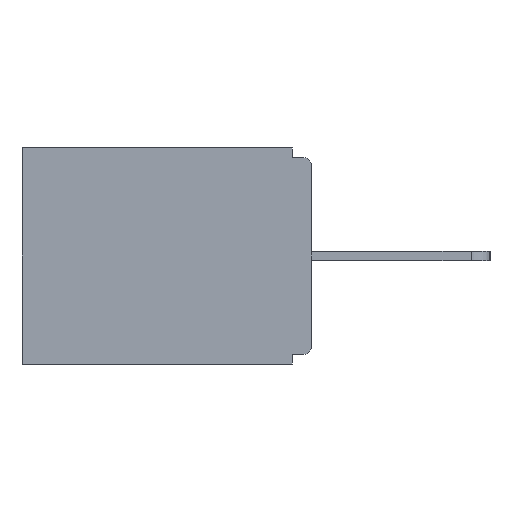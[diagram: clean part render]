
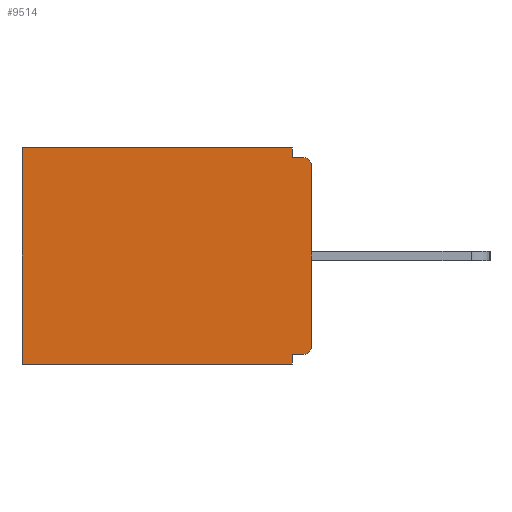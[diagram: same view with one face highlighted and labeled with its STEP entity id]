
A CAD part, left-side view. The second image highlights one B-rep face of the part: STEP entity #9514.
In plain terms, the highlighted planar face has unit normal (-1, 0, 0).
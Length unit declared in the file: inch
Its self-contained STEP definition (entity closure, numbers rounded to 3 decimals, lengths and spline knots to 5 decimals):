
#617 = VECTOR ( 'NONE', #4318, 39.37008 ) ;
#638 = CARTESIAN_POINT ( 'NONE',  ( 0.298, 0.015, -0.015 ) ) ;
#838 = EDGE_CURVE ( 'NONE', #17202, #10318, #16039, .T. ) ;
#1009 = ORIENTED_EDGE ( 'NONE', *, *, #4392, .F. ) ;
#1059 = CARTESIAN_POINT ( 'NONE',  ( 0.298, 0., -0.328 ) ) ;
#1076 = ORIENTED_EDGE ( 'NONE', *, *, #10512, .T. ) ;
#1226 = DIRECTION ( 'NONE',  ( 0., 0., -1. ) ) ;
#1297 = CARTESIAN_POINT ( 'NONE',  ( 0.298, 0.015, -0.03 ) ) ;
#1445 = CARTESIAN_POINT ( 'NONE',  ( 0.298, 0.015, -0.328 ) ) ;
#1468 = VERTEX_POINT ( 'NONE', #1445 ) ;
#1560 = EDGE_CURVE ( 'NONE', #2902, #17478, #16222, .T. ) ;
#1816 = DIRECTION ( 'NONE',  ( -1., 0., 0. ) ) ;
#1899 = ORIENTED_EDGE ( 'NONE', *, *, #18720, .T. ) ;
#2090 = CARTESIAN_POINT ( 'NONE',  ( 0.298, 0., -0.03 ) ) ;
#2370 = FACE_OUTER_BOUND ( 'NONE', #15454, .T. ) ;
#2758 = CARTESIAN_POINT ( 'NONE',  ( 0.298, 0.031, -0.015 ) ) ;
#2902 = VERTEX_POINT ( 'NONE', #5034 ) ;
#3115 = CARTESIAN_POINT ( 'NONE',  ( 0.298, 0., 0. ) ) ;
#3401 = LINE ( 'NONE', #1059, #6909 ) ;
#3741 = CIRCLE ( 'NONE', #11944, 0.015 ) ;
#3927 = VECTOR ( 'NONE', #10064, 39.37008 ) ;
#4150 = AXIS2_PLACEMENT_3D ( 'NONE', #5391, #15272, #15262 ) ;
#4168 = CARTESIAN_POINT ( 'NONE',  ( 0.298, 0., -0.313 ) ) ;
#4318 = DIRECTION ( 'NONE',  ( 0., 1., 0. ) ) ;
#4392 = EDGE_CURVE ( 'NONE', #17833, #2902, #10029, .T. ) ;
#4540 = VECTOR ( 'NONE', #6418, 39.37008 ) ;
#4800 = ORIENTED_EDGE ( 'NONE', *, *, #838, .F. ) ;
#4838 = VERTEX_POINT ( 'NONE', #2090 ) ;
#5034 = CARTESIAN_POINT ( 'NONE',  ( 0.298, 0.031, -0.343 ) ) ;
#5391 = CARTESIAN_POINT ( 'NONE',  ( 0.298, 0., 0. ) ) ;
#5638 = CARTESIAN_POINT ( 'NONE',  ( 0.298, 0.46, 0. ) ) ;
#6418 = DIRECTION ( 'NONE',  ( 0., 1., 0. ) ) ;
#6713 = DIRECTION ( 'NONE',  ( 0., -1., 0. ) ) ;
#6909 = VECTOR ( 'NONE', #8529, 39.37008 ) ;
#6926 = ORIENTED_EDGE ( 'NONE', *, *, #1560, .F. ) ;
#7310 = EDGE_CURVE ( 'NONE', #13010, #17202, #8992, .T. ) ;
#8517 = VECTOR ( 'NONE', #13538, 39.37008 ) ;
#8529 = DIRECTION ( 'NONE',  ( 0., 1., 0. ) ) ;
#8587 = CARTESIAN_POINT ( 'NONE',  ( 0.298, 0.46, 0. ) ) ;
#8992 = LINE ( 'NONE', #16313, #8517 ) ;
#9303 = ORIENTED_EDGE ( 'NONE', *, *, #17998, .F. ) ;
#9337 = ORIENTED_EDGE ( 'NONE', *, *, #9450, .T. ) ;
#9421 = ORIENTED_EDGE ( 'NONE', *, *, #7310, .F. ) ;
#9450 = EDGE_CURVE ( 'NONE', #1468, #17165, #14563, .T. ) ;
#9514 = ADVANCED_FACE ( 'NONE', ( #2370 ), #13501, .F. ) ;
#10029 = LINE ( 'NONE', #14593, #16777 ) ;
#10064 = DIRECTION ( 'NONE',  ( 0., 0., -1. ) ) ;
#10276 = DIRECTION ( 'NONE',  ( 0., 0., -1. ) ) ;
#10318 = VERTEX_POINT ( 'NONE', #638 ) ;
#10512 = EDGE_CURVE ( 'NONE', #4838, #10318, #3741, .T. ) ;
#10717 = CARTESIAN_POINT ( 'NONE',  ( 0.298, 0.46, -0.343 ) ) ;
#11944 = AXIS2_PLACEMENT_3D ( 'NONE', #1297, #1816, #1226 ) ;
#12176 = VECTOR ( 'NONE', #6713, 39.37008 ) ;
#12226 = LINE ( 'NONE', #8587, #3927 ) ;
#12378 = DIRECTION ( 'NONE',  ( 0., 0., -1. ) ) ;
#12394 = DIRECTION ( 'NONE',  ( -1., 0., 0. ) ) ;
#12439 = CARTESIAN_POINT ( 'NONE',  ( 0.298, 0.015, -0.313 ) ) ;
#12443 = LINE ( 'NONE', #13131, #617 ) ;
#12695 = VECTOR ( 'NONE', #14874, 39.37008 ) ;
#12780 = EDGE_CURVE ( 'NONE', #18657, #17478, #12226, .T. ) ;
#13010 = VERTEX_POINT ( 'NONE', #17733 ) ;
#13131 = CARTESIAN_POINT ( 'NONE',  ( 0.298, 0., 0. ) ) ;
#13501 = PLANE ( 'NONE',  #4150 ) ;
#13538 = DIRECTION ( 'NONE',  ( 0., 0., -1. ) ) ;
#13609 = LINE ( 'NONE', #3115, #12695 ) ;
#14363 = CARTESIAN_POINT ( 'NONE',  ( 0.298, 0.031, -0.328 ) ) ;
#14369 = AXIS2_PLACEMENT_3D ( 'NONE', #12439, #12394, #12378 ) ;
#14563 = CIRCLE ( 'NONE', #14369, 0.015 ) ;
#14593 = CARTESIAN_POINT ( 'NONE',  ( 0.298, 0.031, -0.343 ) ) ;
#14597 = EDGE_CURVE ( 'NONE', #1468, #17833, #3401, .T. ) ;
#14874 = DIRECTION ( 'NONE',  ( 0., 0., -1. ) ) ;
#15262 = DIRECTION ( 'NONE',  ( 0., 0., -1. ) ) ;
#15272 = DIRECTION ( 'NONE',  ( 1., 0., 0. ) ) ;
#15454 = EDGE_LOOP ( 'NONE', ( #1076, #4800, #9421, #1899, #18957, #6926, #1009, #18369, #9337, #9303 ) ) ;
#16039 = LINE ( 'NONE', #16282, #12176 ) ;
#16222 = LINE ( 'NONE', #17735, #4540 ) ;
#16282 = CARTESIAN_POINT ( 'NONE',  ( 0.298, 0., -0.015 ) ) ;
#16313 = CARTESIAN_POINT ( 'NONE',  ( 0.298, 0.031, -0.343 ) ) ;
#16777 = VECTOR ( 'NONE', #10276, 39.37008 ) ;
#17165 = VERTEX_POINT ( 'NONE', #4168 ) ;
#17202 = VERTEX_POINT ( 'NONE', #2758 ) ;
#17478 = VERTEX_POINT ( 'NONE', #10717 ) ;
#17733 = CARTESIAN_POINT ( 'NONE',  ( 0.298, 0.031, 0. ) ) ;
#17735 = CARTESIAN_POINT ( 'NONE',  ( 0.298, 0., -0.343 ) ) ;
#17833 = VERTEX_POINT ( 'NONE', #14363 ) ;
#17998 = EDGE_CURVE ( 'NONE', #4838, #17165, #13609, .T. ) ;
#18369 = ORIENTED_EDGE ( 'NONE', *, *, #14597, .F. ) ;
#18657 = VERTEX_POINT ( 'NONE', #5638 ) ;
#18720 = EDGE_CURVE ( 'NONE', #13010, #18657, #12443, .T. ) ;
#18957 = ORIENTED_EDGE ( 'NONE', *, *, #12780, .T. ) ;
